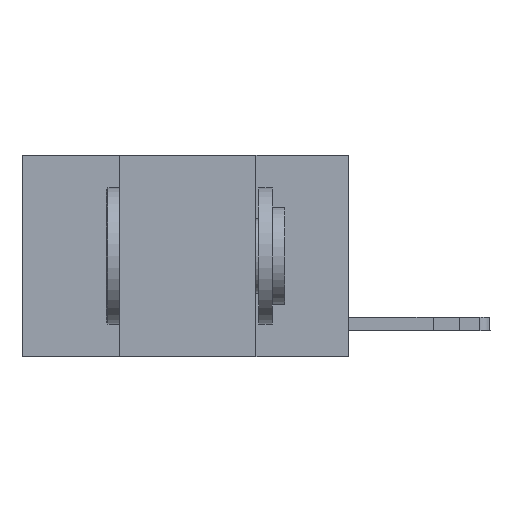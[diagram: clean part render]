
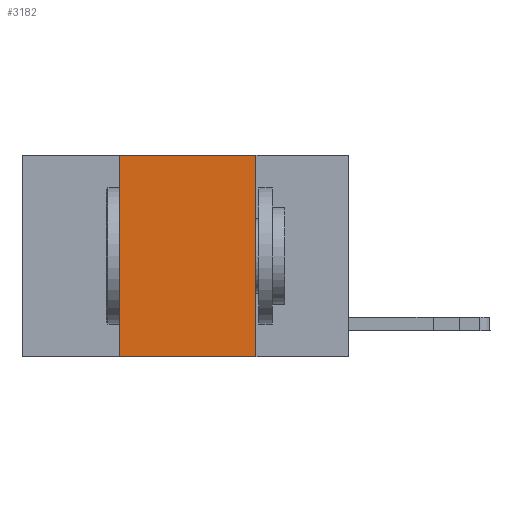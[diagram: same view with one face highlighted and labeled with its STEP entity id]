
A CAD part, left-side view. The second image highlights one B-rep face of the part: STEP entity #3182.
In plain terms, the highlighted planar face has unit normal (-1, 0, 0).
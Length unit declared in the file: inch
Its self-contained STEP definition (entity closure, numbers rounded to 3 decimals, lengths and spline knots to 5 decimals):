
#132 = EDGE_CURVE ( 'NONE', #6276, #6491, #12880, .T. ) ;
#237 = CARTESIAN_POINT ( 'NONE',  ( 0., 0.42, 0. ) ) ;
#552 = EDGE_CURVE ( 'NONE', #7709, #6610, #1458, .T. ) ;
#589 = EDGE_CURVE ( 'NONE', #7709, #6491, #3691, .T. ) ;
#754 = VECTOR ( 'NONE', #10988, 39.37008 ) ;
#815 = CARTESIAN_POINT ( 'NONE',  ( 0., 0.42, 0. ) ) ;
#1216 = CARTESIAN_POINT ( 'NONE',  ( 0., 0.17, 0. ) ) ;
#1458 = LINE ( 'NONE', #237, #6534 ) ;
#2001 = DIRECTION ( 'NONE',  ( 0., 0., -1. ) ) ;
#2031 = CARTESIAN_POINT ( 'NONE',  ( 0., 0.6, 0. ) ) ;
#2436 = LINE ( 'NONE', #2031, #12661 ) ;
#2453 = DIRECTION ( 'NONE',  ( 1., 0., 0. ) ) ;
#2664 = PLANE ( 'NONE',  #12268 ) ;
#3182 = ADVANCED_FACE ( 'NONE', ( #7815 ), #2664, .F. ) ;
#3394 = CARTESIAN_POINT ( 'NONE',  ( 0., 0.6, 0. ) ) ;
#3691 = LINE ( 'NONE', #4681, #754 ) ;
#4186 = DIRECTION ( 'NONE',  ( 0., 0., -1. ) ) ;
#4198 = CARTESIAN_POINT ( 'NONE',  ( 0., 0.17, 0. ) ) ;
#4681 = CARTESIAN_POINT ( 'NONE',  ( 0., 0.6, -0.37 ) ) ;
#5393 = CARTESIAN_POINT ( 'NONE',  ( 0., 0.42, -0.37 ) ) ;
#6276 = VERTEX_POINT ( 'NONE', #1216 ) ;
#6491 = VERTEX_POINT ( 'NONE', #9648 ) ;
#6534 = VECTOR ( 'NONE', #11165, 39.37008 ) ;
#6610 = VERTEX_POINT ( 'NONE', #815 ) ;
#6701 = ORIENTED_EDGE ( 'NONE', *, *, #552, .F. ) ;
#7709 = VERTEX_POINT ( 'NONE', #5393 ) ;
#7815 = FACE_OUTER_BOUND ( 'NONE', #9553, .T. ) ;
#9553 = EDGE_LOOP ( 'NONE', ( #12760, #13615, #6701, #13646 ) ) ;
#9648 = CARTESIAN_POINT ( 'NONE',  ( 0., 0.17, -0.37 ) ) ;
#10988 = DIRECTION ( 'NONE',  ( 0., -1., 0. ) ) ;
#11165 = DIRECTION ( 'NONE',  ( 0., 0., 1. ) ) ;
#11597 = DIRECTION ( 'NONE',  ( 0., -1., 0. ) ) ;
#12268 = AXIS2_PLACEMENT_3D ( 'NONE', #3394, #2453, #2001 ) ;
#12661 = VECTOR ( 'NONE', #11597, 39.37008 ) ;
#12760 = ORIENTED_EDGE ( 'NONE', *, *, #132, .F. ) ;
#12880 = LINE ( 'NONE', #4198, #13198 ) ;
#12887 = EDGE_CURVE ( 'NONE', #6610, #6276, #2436, .T. ) ;
#13198 = VECTOR ( 'NONE', #4186, 39.37008 ) ;
#13615 = ORIENTED_EDGE ( 'NONE', *, *, #12887, .F. ) ;
#13646 = ORIENTED_EDGE ( 'NONE', *, *, #589, .T. ) ;
